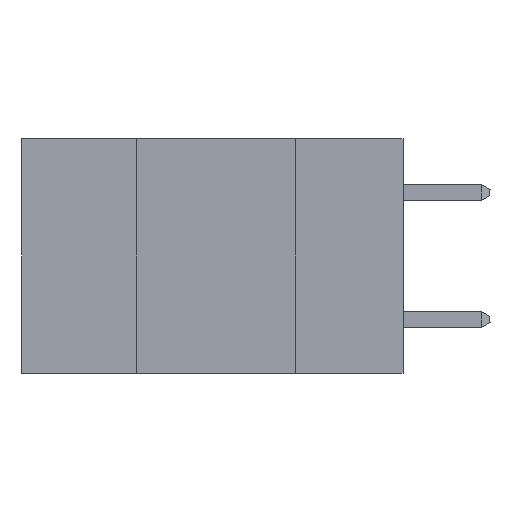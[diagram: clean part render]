
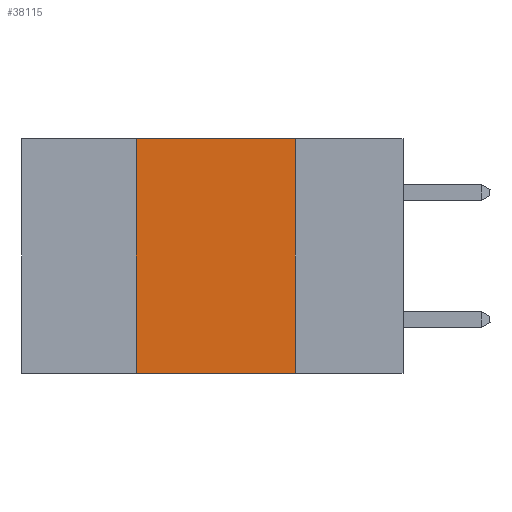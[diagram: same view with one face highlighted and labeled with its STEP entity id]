
A CAD part, left-side view. The second image highlights one B-rep face of the part: STEP entity #38115.
In plain terms, the highlighted planar face has unit normal (-1, 0, 0).
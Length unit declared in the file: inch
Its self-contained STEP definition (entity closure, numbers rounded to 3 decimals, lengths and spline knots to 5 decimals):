
#603 = ORIENTED_EDGE ( 'NONE', *, *, #1836, .T. ) ;
#1836 = EDGE_CURVE ( 'NONE', #41948, #39675, #36041, .T. ) ;
#4583 = DIRECTION ( 'NONE',  ( 0., 0., -1. ) ) ;
#5997 = EDGE_CURVE ( 'NONE', #21902, #6662, #33187, .T. ) ;
#6281 = CARTESIAN_POINT ( 'NONE',  ( 0., 0.6, -0.37 ) ) ;
#6662 = VERTEX_POINT ( 'NONE', #21236 ) ;
#7113 = AXIS2_PLACEMENT_3D ( 'NONE', #39170, #50296, #38673 ) ;
#7448 = PLANE ( 'NONE',  #7113 ) ;
#10101 = EDGE_CURVE ( 'NONE', #6662, #39675, #48445, .T. ) ;
#13078 = EDGE_LOOP ( 'NONE', ( #17073, #47473, #46687, #603 ) ) ;
#15991 = CARTESIAN_POINT ( 'NONE',  ( 0., 0.17, -0.37 ) ) ;
#17073 = ORIENTED_EDGE ( 'NONE', *, *, #10101, .F. ) ;
#18126 = LINE ( 'NONE', #38652, #37984 ) ;
#20418 = CARTESIAN_POINT ( 'NONE',  ( 0., 0.17, 0. ) ) ;
#21236 = CARTESIAN_POINT ( 'NONE',  ( 0., 0.17, 0. ) ) ;
#21902 = VERTEX_POINT ( 'NONE', #36705 ) ;
#22924 = DIRECTION ( 'NONE',  ( 0., 0., 1. ) ) ;
#23054 = VECTOR ( 'NONE', #30239, 39.37008 ) ;
#25190 = EDGE_CURVE ( 'NONE', #41948, #21902, #18126, .T. ) ;
#28918 = DIRECTION ( 'NONE',  ( 0., -1., 0. ) ) ;
#29376 = FACE_OUTER_BOUND ( 'NONE', #13078, .T. ) ;
#29423 = CARTESIAN_POINT ( 'NONE',  ( 0., 0.6, 0. ) ) ;
#30138 = CARTESIAN_POINT ( 'NONE',  ( 0., 0.42, -0.37 ) ) ;
#30239 = DIRECTION ( 'NONE',  ( 0., -1., 0. ) ) ;
#33187 = LINE ( 'NONE', #29423, #48036 ) ;
#36041 = LINE ( 'NONE', #6281, #23054 ) ;
#36705 = CARTESIAN_POINT ( 'NONE',  ( 0., 0.42, 0. ) ) ;
#37894 = VECTOR ( 'NONE', #4583, 39.37008 ) ;
#37984 = VECTOR ( 'NONE', #22924, 39.37008 ) ;
#38115 = ADVANCED_FACE ( 'NONE', ( #29376 ), #7448, .F. ) ;
#38652 = CARTESIAN_POINT ( 'NONE',  ( 0., 0.42, 0. ) ) ;
#38673 = DIRECTION ( 'NONE',  ( 0., 0., -1. ) ) ;
#39170 = CARTESIAN_POINT ( 'NONE',  ( 0., 0.6, 0. ) ) ;
#39675 = VERTEX_POINT ( 'NONE', #15991 ) ;
#41948 = VERTEX_POINT ( 'NONE', #30138 ) ;
#46687 = ORIENTED_EDGE ( 'NONE', *, *, #25190, .F. ) ;
#47473 = ORIENTED_EDGE ( 'NONE', *, *, #5997, .F. ) ;
#48036 = VECTOR ( 'NONE', #28918, 39.37008 ) ;
#48445 = LINE ( 'NONE', #20418, #37894 ) ;
#50296 = DIRECTION ( 'NONE',  ( 1., 0., 0. ) ) ;
